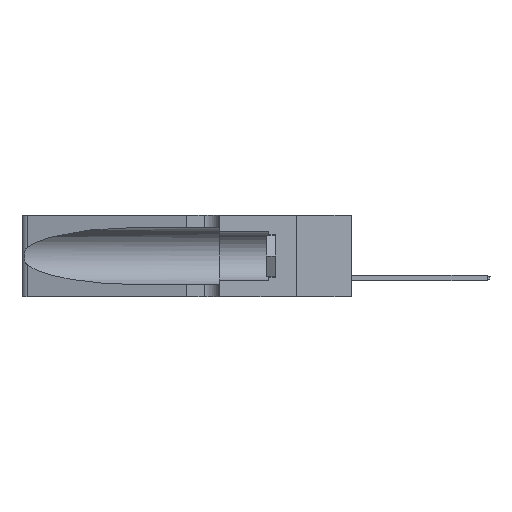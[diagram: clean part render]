
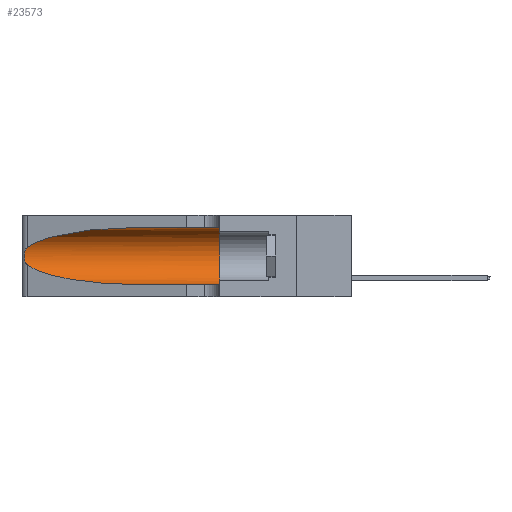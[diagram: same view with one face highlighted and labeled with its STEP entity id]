
A CAD part, left-side view. The second image highlights one B-rep face of the part: STEP entity #23573.
In plain terms, the highlighted cylindrical face has radius 3.308 mm (diameter 6.617 mm), a partial arc.
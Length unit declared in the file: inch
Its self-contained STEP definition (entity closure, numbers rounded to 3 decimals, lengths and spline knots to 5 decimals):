
#71 = CARTESIAN_POINT ( 'NONE',  ( 0.1305, 1.61858, 0.05475 ) ) ;
#269 =( BOUNDED_CURVE ( )  B_SPLINE_CURVE ( 3, ( #16428, #21659, #19672, #5803 ),
 .UNSPECIFIED., .F., .T. ) 
 B_SPLINE_CURVE_WITH_KNOTS ( ( 4, 4 ),
 ( 3.44316, 4.71239 ),
 .UNSPECIFIED. ) 
 CURVE ( )  GEOMETRIC_REPRESENTATION_ITEM ( )  RATIONAL_B_SPLINE_CURVE ( ( 1., 0.87, 0.87, 1. ) ) 
 REPRESENTATION_ITEM ( '' )  );
#900 = CARTESIAN_POINT ( 'NONE',  ( 0.18966, 0.96281, 0.31525 ) ) ;
#1286 = EDGE_CURVE ( 'NONE', #16180, #32904, #269, .T. ) ;
#1401 = DIRECTION ( 'NONE',  ( 0., 1., 0. ) ) ;
#1525 = CARTESIAN_POINT ( 'NONE',  ( 0.25854, 1.2359, 0.20912 ) ) ;
#1672 = EDGE_CURVE ( 'NONE', #32904, #30481, #4881, .T. ) ;
#1697 = EDGE_CURVE ( 'NONE', #11293, #30481, #12648, .T. ) ;
#2359 = CARTESIAN_POINT ( 'NONE',  ( 0.25487, 1.22718, 0.14631 ) ) ;
#3758 = AXIS2_PLACEMENT_3D ( 'NONE', #31823, #1401, #23318 ) ;
#4395 = CARTESIAN_POINT ( 'NONE',  ( 0.26017, 1.23833, 0.17102 ) ) ;
#4881 = LINE ( 'NONE', #71, #19061 ) ;
#5341 = EDGE_CURVE ( 'NONE', #6259, #16180, #29692, .T. ) ;
#5694 = ORIENTED_EDGE ( 'NONE', *, *, #23923, .F. ) ;
#5803 = CARTESIAN_POINT ( 'NONE',  ( 0.1305, 0.72297, 0.05475 ) ) ;
#6259 = VERTEX_POINT ( 'NONE', #21837 ) ;
#6737 = ORIENTED_EDGE ( 'NONE', *, *, #1697, .F. ) ;
#6832 = ORIENTED_EDGE ( 'NONE', *, *, #1286, .T. ) ;
#7618 = DIRECTION ( 'NONE',  ( 0., 0., -1. ) ) ;
#8288 = DIRECTION ( 'NONE',  ( 0., -1., 0. ) ) ;
#8517 = LINE ( 'NONE', #8721, #14958 ) ;
#8721 = CARTESIAN_POINT ( 'NONE',  ( 0.1305, 1.61858, 0.31525 ) ) ;
#10095 = CARTESIAN_POINT ( 'NONE',  ( 0.25639, 1.23184, 0.21858 ) ) ;
#11293 = VERTEX_POINT ( 'NONE', #24082 ) ;
#12648 = CIRCLE ( 'NONE', #3758, 0.13025 ) ;
#12864 = CARTESIAN_POINT ( 'NONE',  ( 0.25787, 1.23484, 0.2124 ) ) ;
#13420 = CARTESIAN_POINT ( 'NONE',  ( 0.1305, 0.72297, 0.31525 ) ) ;
#13793 = CARTESIAN_POINT ( 'NONE',  ( 0.1305, 0.72297, 0.05475 ) ) ;
#14352 = DIRECTION ( 'NONE',  ( 0., -1., 0. ) ) ;
#14924 = VERTEX_POINT ( 'NONE', #13420 ) ;
#14958 = VECTOR ( 'NONE', #14352, 39.37008 ) ;
#15644 = DIRECTION ( 'NONE',  ( 0., -1., 0. ) ) ;
#16060 = CARTESIAN_POINT ( 'NONE',  ( 0.25639, 1.23186, 0.15144 ) ) ;
#16180 = VERTEX_POINT ( 'NONE', #20104 ) ;
#16428 = CARTESIAN_POINT ( 'NONE',  ( 0.25487, 1.22718, 0.14631 ) ) ;
#17011 = CARTESIAN_POINT ( 'NONE',  ( 0.25487, 1.22718, 0.22369 ) ) ;
#18134 = CARTESIAN_POINT ( 'NONE',  ( 0.26075, 1.23896, 0.178 ) ) ;
#18585 = ORIENTED_EDGE ( 'NONE', *, *, #5341, .T. ) ;
#19061 = VECTOR ( 'NONE', #8288, 39.37008 ) ;
#19297 = EDGE_CURVE ( 'NONE', #14924, #6259, #33353, .T. ) ;
#19672 = CARTESIAN_POINT ( 'NONE',  ( 0.18966, 0.96281, 0.05475 ) ) ;
#19948 = EDGE_LOOP ( 'NONE', ( #33800, #18585, #6832, #23825, #6737, #5694 ) ) ;
#20104 = CARTESIAN_POINT ( 'NONE',  ( 0.25487, 1.22718, 0.14631 ) ) ;
#20974 = CARTESIAN_POINT ( 'NONE',  ( 0.1305, 1.61858, 0.185 ) ) ;
#21659 = CARTESIAN_POINT ( 'NONE',  ( 0.2373, 1.15595, 0.08982 ) ) ;
#21837 = CARTESIAN_POINT ( 'NONE',  ( 0.25487, 1.22718, 0.22369 ) ) ;
#22942 = CARTESIAN_POINT ( 'NONE',  ( 0.2373, 1.15595, 0.28018 ) ) ;
#23318 = DIRECTION ( 'NONE',  ( 0., 0., 1. ) ) ;
#23435 = CARTESIAN_POINT ( 'NONE',  ( 0.25487, 1.22718, 0.22369 ) ) ;
#23573 = ADVANCED_FACE ( 'NONE', ( #23631 ), #32638, .F. ) ;
#23631 = FACE_OUTER_BOUND ( 'NONE', #19948, .T. ) ;
#23676 = CARTESIAN_POINT ( 'NONE',  ( 0.25856, 1.23593, 0.16098 ) ) ;
#23825 = ORIENTED_EDGE ( 'NONE', *, *, #1672, .T. ) ;
#23923 = EDGE_CURVE ( 'NONE', #14924, #11293, #8517, .T. ) ;
#24082 = CARTESIAN_POINT ( 'NONE',  ( 0.1305, 0.35, 0.31525 ) ) ;
#27139 = CARTESIAN_POINT ( 'NONE',  ( 0.25555, 1.22993, 0.14849 ) ) ;
#29692 = B_SPLINE_CURVE_WITH_KNOTS ( 'NONE', 3,
 ( #23435, #31938, #10095, #12864, #1525, #31819, #34593, #18134, #4395, #23676, #32524, #16060, #27139, #2359 ),
 .UNSPECIFIED., .F., .F.,
 ( 4, 2, 2, 2, 2, 2, 4 ),
 ( 0., 0.00027, 0.00053, 0.00107, 0.0016, 0.00187, 0.00214 ),
 .UNSPECIFIED. ) ;
#30481 = VERTEX_POINT ( 'NONE', #34787 ) ;
#31819 = CARTESIAN_POINT ( 'NONE',  ( 0.26018, 1.23835, 0.19895 ) ) ;
#31823 = CARTESIAN_POINT ( 'NONE',  ( 0.1305, 0.35, 0.185 ) ) ;
#31938 = CARTESIAN_POINT ( 'NONE',  ( 0.25555, 1.22994, 0.2215 ) ) ;
#32524 = CARTESIAN_POINT ( 'NONE',  ( 0.25789, 1.23486, 0.15765 ) ) ;
#32638 = CYLINDRICAL_SURFACE ( 'NONE', #34615, 0.13025 ) ;
#32904 = VERTEX_POINT ( 'NONE', #13793 ) ;
#33353 =( BOUNDED_CURVE ( )  B_SPLINE_CURVE ( 3, ( #33472, #900, #22942, #17011 ),
 .UNSPECIFIED., .F., .F. ) 
 B_SPLINE_CURVE_WITH_KNOTS ( ( 4, 4 ),
 ( 1.5708, 2.84003 ),
 .UNSPECIFIED. ) 
 CURVE ( )  GEOMETRIC_REPRESENTATION_ITEM ( )  RATIONAL_B_SPLINE_CURVE ( ( 1., 0.87, 0.87, 1. ) ) 
 REPRESENTATION_ITEM ( '' )  );
#33472 = CARTESIAN_POINT ( 'NONE',  ( 0.1305, 0.72297, 0.31525 ) ) ;
#33800 = ORIENTED_EDGE ( 'NONE', *, *, #19297, .T. ) ;
#34593 = CARTESIAN_POINT ( 'NONE',  ( 0.26075, 1.23896, 0.19203 ) ) ;
#34615 = AXIS2_PLACEMENT_3D ( 'NONE', #20974, #15644, #7618 ) ;
#34787 = CARTESIAN_POINT ( 'NONE',  ( 0.1305, 0.35, 0.05475 ) ) ;
